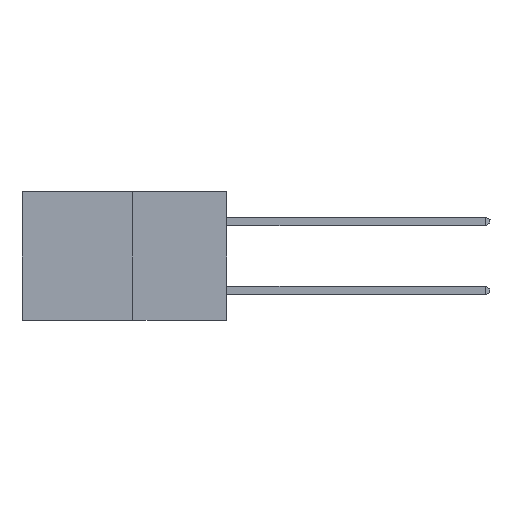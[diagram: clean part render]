
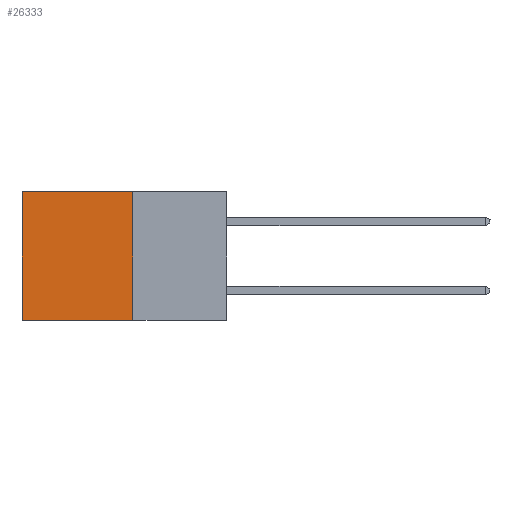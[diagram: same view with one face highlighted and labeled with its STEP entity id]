
A CAD part, left-side view. The second image highlights one B-rep face of the part: STEP entity #26333.
In plain terms, the highlighted planar face has unit normal (-1, 0, 0).
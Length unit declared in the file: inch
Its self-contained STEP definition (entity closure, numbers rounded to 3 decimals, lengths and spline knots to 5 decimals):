
#389 = DIRECTION ( 'NONE',  ( 1., 0., 0. ) ) ;
#1065 = LINE ( 'NONE', #15810, #19329 ) ;
#1514 = AXIS2_PLACEMENT_3D ( 'NONE', #15296, #389, #17811 ) ;
#1549 = EDGE_CURVE ( 'NONE', #6016, #4964, #18528, .T. ) ;
#2121 = FACE_OUTER_BOUND ( 'NONE', #27422, .T. ) ;
#2917 = CARTESIAN_POINT ( 'NONE',  ( 0.277, 0.59, -0.37 ) ) ;
#3289 = ORIENTED_EDGE ( 'NONE', *, *, #1549, .T. ) ;
#3519 = DIRECTION ( 'NONE',  ( 0., 1., 0. ) ) ;
#4777 = DIRECTION ( 'NONE',  ( 0., 0., -1. ) ) ;
#4964 = VERTEX_POINT ( 'NONE', #13647 ) ;
#6016 = VERTEX_POINT ( 'NONE', #20383 ) ;
#6974 = ORIENTED_EDGE ( 'NONE', *, *, #29553, .F. ) ;
#7368 = CARTESIAN_POINT ( 'NONE',  ( 0.277, 0.27, 0. ) ) ;
#9237 = VECTOR ( 'NONE', #4777, 39.37008 ) ;
#13647 = CARTESIAN_POINT ( 'NONE',  ( 0.277, 0.59, -0.37 ) ) ;
#13769 = CARTESIAN_POINT ( 'NONE',  ( 0.277, 0.27, 0. ) ) ;
#14647 = ORIENTED_EDGE ( 'NONE', *, *, #23898, .F. ) ;
#15296 = CARTESIAN_POINT ( 'NONE',  ( 0.277, 0.27, -0.37 ) ) ;
#15792 = LINE ( 'NONE', #22043, #9237 ) ;
#15797 = CARTESIAN_POINT ( 'NONE',  ( 0.277, 0.27, -0.37 ) ) ;
#15810 = CARTESIAN_POINT ( 'NONE',  ( 0.277, 0.27, -0.37 ) ) ;
#16188 = ORIENTED_EDGE ( 'NONE', *, *, #26595, .T. ) ;
#17811 = DIRECTION ( 'NONE',  ( 0., 0., -1. ) ) ;
#18528 = LINE ( 'NONE', #2917, #30774 ) ;
#19329 = VECTOR ( 'NONE', #3519, 39.37008 ) ;
#20383 = CARTESIAN_POINT ( 'NONE',  ( 0.277, 0.59, 0. ) ) ;
#20554 = DIRECTION ( 'NONE',  ( 0., 0., -1. ) ) ;
#20697 = VECTOR ( 'NONE', #26054, 39.37008 ) ;
#22043 = CARTESIAN_POINT ( 'NONE',  ( 0.277, 0.27, -0.37 ) ) ;
#23898 = EDGE_CURVE ( 'NONE', #25200, #4964, #1065, .T. ) ;
#25200 = VERTEX_POINT ( 'NONE', #15797 ) ;
#25639 = VERTEX_POINT ( 'NONE', #7368 ) ;
#26054 = DIRECTION ( 'NONE',  ( 0., 1., 0. ) ) ;
#26333 = ADVANCED_FACE ( 'NONE', ( #2121 ), #27550, .F. ) ;
#26595 = EDGE_CURVE ( 'NONE', #25639, #6016, #27190, .T. ) ;
#27190 = LINE ( 'NONE', #13769, #20697 ) ;
#27422 = EDGE_LOOP ( 'NONE', ( #3289, #14647, #6974, #16188 ) ) ;
#27550 = PLANE ( 'NONE',  #1514 ) ;
#29553 = EDGE_CURVE ( 'NONE', #25639, #25200, #15792, .T. ) ;
#30774 = VECTOR ( 'NONE', #20554, 39.37008 ) ;
